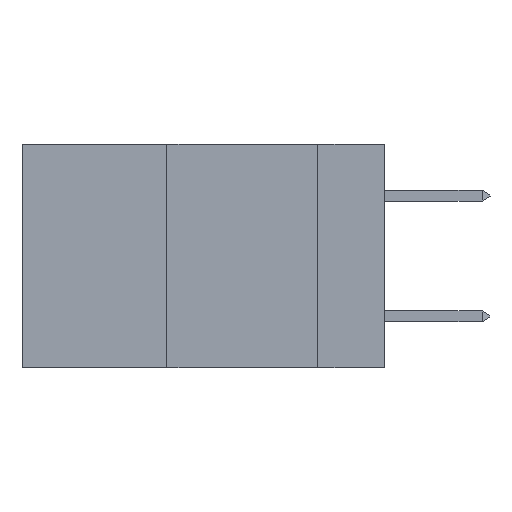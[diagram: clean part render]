
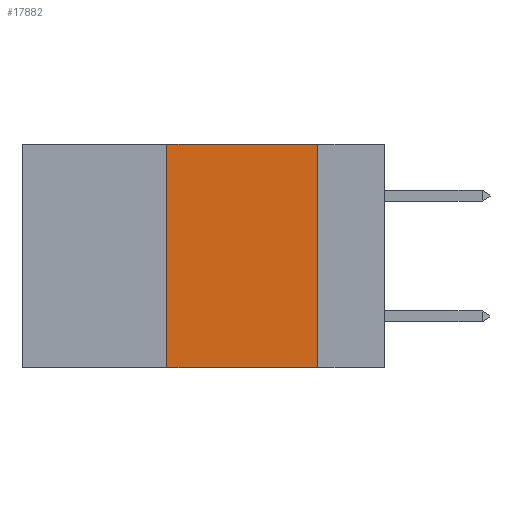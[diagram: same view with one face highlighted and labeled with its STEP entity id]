
A CAD part, left-side view. The second image highlights one B-rep face of the part: STEP entity #17882.
In plain terms, the highlighted planar face has unit normal (-1, 0, 0).
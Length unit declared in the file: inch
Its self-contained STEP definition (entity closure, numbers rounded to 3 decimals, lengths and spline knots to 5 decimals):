
#36 = EDGE_LOOP ( 'NONE', ( #12476, #7048, #13140, #14129 ) ) ;
#1089 = CARTESIAN_POINT ( 'NONE',  ( 0., 0.36, -0.37 ) ) ;
#1892 = CARTESIAN_POINT ( 'NONE',  ( 0., 0.6, 0. ) ) ;
#1953 = VECTOR ( 'NONE', #3715, 39.37008 ) ;
#2886 = AXIS2_PLACEMENT_3D ( 'NONE', #14178, #6120, #17077 ) ;
#3401 = CARTESIAN_POINT ( 'NONE',  ( 0., 0.11, 0. ) ) ;
#3715 = DIRECTION ( 'NONE',  ( 0., -1., 0. ) ) ;
#3717 = VECTOR ( 'NONE', #17725, 39.37008 ) ;
#4657 = FACE_OUTER_BOUND ( 'NONE', #36, .T. ) ;
#6120 = DIRECTION ( 'NONE',  ( 1., 0., 0. ) ) ;
#6995 = EDGE_CURVE ( 'NONE', #16332, #15123, #12839, .T. ) ;
#7048 = ORIENTED_EDGE ( 'NONE', *, *, #15842, .F. ) ;
#7870 = DIRECTION ( 'NONE',  ( 0., -1., 0. ) ) ;
#9457 = EDGE_CURVE ( 'NONE', #15499, #15123, #11788, .T. ) ;
#10051 = VERTEX_POINT ( 'NONE', #11701 ) ;
#10172 = DIRECTION ( 'NONE',  ( 0., 0., -1. ) ) ;
#11465 = EDGE_CURVE ( 'NONE', #15499, #10051, #12057, .T. ) ;
#11701 = CARTESIAN_POINT ( 'NONE',  ( 0., 0.36, 0. ) ) ;
#11788 = LINE ( 'NONE', #17630, #16506 ) ;
#12057 = LINE ( 'NONE', #12155, #3717 ) ;
#12155 = CARTESIAN_POINT ( 'NONE',  ( 0., 0.36, 0. ) ) ;
#12265 = CARTESIAN_POINT ( 'NONE',  ( 0., 0.11, 0. ) ) ;
#12476 = ORIENTED_EDGE ( 'NONE', *, *, #6995, .F. ) ;
#12839 = LINE ( 'NONE', #3401, #13127 ) ;
#13127 = VECTOR ( 'NONE', #10172, 39.37008 ) ;
#13140 = ORIENTED_EDGE ( 'NONE', *, *, #11465, .F. ) ;
#13639 = CARTESIAN_POINT ( 'NONE',  ( 0., 0.11, -0.37 ) ) ;
#14129 = ORIENTED_EDGE ( 'NONE', *, *, #9457, .T. ) ;
#14178 = CARTESIAN_POINT ( 'NONE',  ( 0., 0.6, 0. ) ) ;
#14266 = PLANE ( 'NONE',  #2886 ) ;
#15123 = VERTEX_POINT ( 'NONE', #13639 ) ;
#15499 = VERTEX_POINT ( 'NONE', #1089 ) ;
#15770 = LINE ( 'NONE', #1892, #1953 ) ;
#15842 = EDGE_CURVE ( 'NONE', #10051, #16332, #15770, .T. ) ;
#16332 = VERTEX_POINT ( 'NONE', #12265 ) ;
#16506 = VECTOR ( 'NONE', #7870, 39.37008 ) ;
#17077 = DIRECTION ( 'NONE',  ( 0., 0., -1. ) ) ;
#17630 = CARTESIAN_POINT ( 'NONE',  ( 0., 0.6, -0.37 ) ) ;
#17725 = DIRECTION ( 'NONE',  ( 0., 0., 1. ) ) ;
#17882 = ADVANCED_FACE ( 'NONE', ( #4657 ), #14266, .F. ) ;
